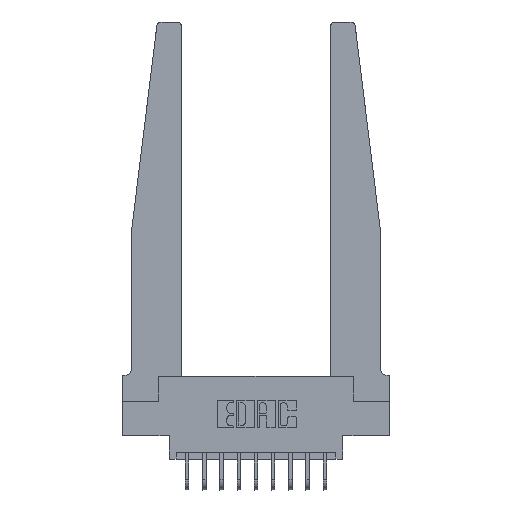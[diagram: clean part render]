
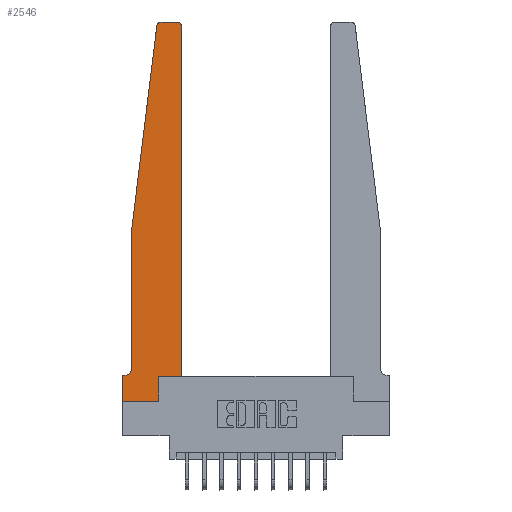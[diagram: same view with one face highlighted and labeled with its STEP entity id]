
A CAD part, top view. The second image highlights one B-rep face of the part: STEP entity #2546.
In plain terms, the highlighted planar face has unit normal (0, 0, 1).
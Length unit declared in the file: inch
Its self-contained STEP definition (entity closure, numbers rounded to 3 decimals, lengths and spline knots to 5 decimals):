
#335 = EDGE_LOOP ( 'NONE', ( #10804, #16728, #8403, #9608, #5358, #16873, #14625, #6112, #15196, #16663, #15041, #6610 ) ) ;
#360 = DIRECTION ( 'NONE',  ( 1., 0., 0. ) ) ;
#439 = DIRECTION ( 'NONE',  ( 0., 0., 1. ) ) ;
#621 = CARTESIAN_POINT ( 'NONE',  ( 0., 0.1875, 0.37 ) ) ;
#931 = EDGE_CURVE ( 'NONE', #7336, #2354, #7570, .T. ) ;
#939 = CARTESIAN_POINT ( 'NONE',  ( 0.065, 1.25, 0.37 ) ) ;
#1289 = VECTOR ( 'NONE', #5804, 39.37008 ) ;
#1539 = CARTESIAN_POINT ( 'NONE',  ( 0.25, 2.75, 0.37 ) ) ;
#1675 = AXIS2_PLACEMENT_3D ( 'NONE', #13910, #439, #15521 ) ;
#1919 = EDGE_CURVE ( 'NONE', #13978, #9623, #15822, .T. ) ;
#2292 = DIRECTION ( 'NONE',  ( 0., 0., -1. ) ) ;
#2296 = CARTESIAN_POINT ( 'NONE',  ( 0.015, 0.1875, 0.37 ) ) ;
#2354 = VERTEX_POINT ( 'NONE', #2296 ) ;
#2460 = EDGE_CURVE ( 'NONE', #5605, #12846, #15492, .T. ) ;
#2537 = DIRECTION ( 'NONE',  ( -0.122, -0.992, 0. ) ) ;
#2546 = ADVANCED_FACE ( 'NONE', ( #13732 ), #3245, .T. ) ;
#2729 = EDGE_CURVE ( 'NONE', #17421, #4041, #17077, .T. ) ;
#2740 = VERTEX_POINT ( 'NONE', #8982 ) ;
#2864 = CARTESIAN_POINT ( 'NONE',  ( 0.2605, 0., 0.37 ) ) ;
#3117 = DIRECTION ( 'NONE',  ( -1., 0., 0. ) ) ;
#3245 = PLANE ( 'NONE',  #6204 ) ;
#3378 = VECTOR ( 'NONE', #5055, 39.37008 ) ;
#3741 = CARTESIAN_POINT ( 'NONE',  ( 0.425, 0.18, 0.37 ) ) ;
#3775 = EDGE_CURVE ( 'NONE', #5778, #13978, #10213, .T. ) ;
#3785 = CARTESIAN_POINT ( 'NONE',  ( 0., 0., 0.37 ) ) ;
#4041 = VERTEX_POINT ( 'NONE', #16283 ) ;
#4111 = DIRECTION ( 'NONE',  ( -1., 0., 0. ) ) ;
#4473 = CARTESIAN_POINT ( 'NONE',  ( 0.395, 2.75, 0.37 ) ) ;
#4482 = CARTESIAN_POINT ( 'NONE',  ( 0.425, 0.18, 0.37 ) ) ;
#5036 = VECTOR ( 'NONE', #10310, 39.37008 ) ;
#5055 = DIRECTION ( 'NONE',  ( 0., -1., 0. ) ) ;
#5325 = EDGE_CURVE ( 'NONE', #12846, #2740, #13802, .T. ) ;
#5356 = VERTEX_POINT ( 'NONE', #14887 ) ;
#5358 = ORIENTED_EDGE ( 'NONE', *, *, #931, .T. ) ;
#5383 = CARTESIAN_POINT ( 'NONE',  ( 0.065, 0.2375, 0.37 ) ) ;
#5605 = VERTEX_POINT ( 'NONE', #11864 ) ;
#5778 = VERTEX_POINT ( 'NONE', #2864 ) ;
#5804 = DIRECTION ( 'NONE',  ( 0., 1., 0. ) ) ;
#5929 = VERTEX_POINT ( 'NONE', #7438 ) ;
#6001 = EDGE_CURVE ( 'NONE', #4041, #7336, #17312, .T. ) ;
#6112 = ORIENTED_EDGE ( 'NONE', *, *, #16059, .T. ) ;
#6204 = AXIS2_PLACEMENT_3D ( 'NONE', #621, #7048, #360 ) ;
#6610 = ORIENTED_EDGE ( 'NONE', *, *, #2460, .T. ) ;
#6832 = CARTESIAN_POINT ( 'NONE',  ( 0.27653, 2.72, 0.37 ) ) ;
#7048 = DIRECTION ( 'NONE',  ( 0., 0., 1. ) ) ;
#7225 = CIRCLE ( 'NONE', #17085, 0.03 ) ;
#7336 = VERTEX_POINT ( 'NONE', #5383 ) ;
#7392 = CARTESIAN_POINT ( 'NONE',  ( 0.425, 0.18, 0.37 ) ) ;
#7438 = CARTESIAN_POINT ( 'NONE',  ( 0., 0., 0.37 ) ) ;
#7570 = CIRCLE ( 'NONE', #8400, 0.05 ) ;
#7676 = DIRECTION ( 'NONE',  ( -1., 0., 0. ) ) ;
#8400 = AXIS2_PLACEMENT_3D ( 'NONE', #10238, #2292, #7676 ) ;
#8403 = ORIENTED_EDGE ( 'NONE', *, *, #2729, .T. ) ;
#8982 = CARTESIAN_POINT ( 'NONE',  ( 0.27653, 2.75, 0.37 ) ) ;
#9178 = VECTOR ( 'NONE', #15874, 39.37008 ) ;
#9466 = DIRECTION ( 'NONE',  ( 0., 0., 1. ) ) ;
#9608 = ORIENTED_EDGE ( 'NONE', *, *, #6001, .T. ) ;
#9623 = VERTEX_POINT ( 'NONE', #4482 ) ;
#9911 = LINE ( 'NONE', #16681, #13357 ) ;
#10213 = LINE ( 'NONE', #14179, #14882 ) ;
#10238 = CARTESIAN_POINT ( 'NONE',  ( 0.015, 0.2375, 0.37 ) ) ;
#10310 = DIRECTION ( 'NONE',  ( 0., -1., 0. ) ) ;
#10499 = CARTESIAN_POINT ( 'NONE',  ( 0., 0., 0.37 ) ) ;
#10608 = CARTESIAN_POINT ( 'NONE',  ( 0.2605, 0.18, 0.37 ) ) ;
#10804 = ORIENTED_EDGE ( 'NONE', *, *, #5325, .T. ) ;
#10983 = VECTOR ( 'NONE', #15564, 39.37008 ) ;
#11339 = EDGE_CURVE ( 'NONE', #5356, #5929, #11895, .T. ) ;
#11864 = CARTESIAN_POINT ( 'NONE',  ( 0.425, 2.72, 0.37 ) ) ;
#11895 = LINE ( 'NONE', #3785, #5036 ) ;
#11939 = DIRECTION ( 'NONE',  ( 1., 0., 0. ) ) ;
#12330 = CARTESIAN_POINT ( 'NONE',  ( 0.24675, 2.72367, 0.37 ) ) ;
#12846 = VERTEX_POINT ( 'NONE', #4473 ) ;
#12855 = LINE ( 'NONE', #7392, #1289 ) ;
#13004 = CARTESIAN_POINT ( 'NONE',  ( 0.065, 1.25, 0.37 ) ) ;
#13357 = VECTOR ( 'NONE', #3117, 39.37008 ) ;
#13712 = EDGE_CURVE ( 'NONE', #2354, #5356, #9911, .T. ) ;
#13732 = FACE_OUTER_BOUND ( 'NONE', #335, .T. ) ;
#13781 = VECTOR ( 'NONE', #2537, 39.37008 ) ;
#13802 = LINE ( 'NONE', #1539, #17190 ) ;
#13910 = CARTESIAN_POINT ( 'NONE',  ( 0.395, 2.72, 0.37 ) ) ;
#13978 = VERTEX_POINT ( 'NONE', #10608 ) ;
#14179 = CARTESIAN_POINT ( 'NONE',  ( 0.2605, 0.18, 0.37 ) ) ;
#14359 = DIRECTION ( 'NONE',  ( 0., 1., 0. ) ) ;
#14625 = ORIENTED_EDGE ( 'NONE', *, *, #11339, .T. ) ;
#14882 = VECTOR ( 'NONE', #14359, 39.37008 ) ;
#14887 = CARTESIAN_POINT ( 'NONE',  ( 0., 0.1875, 0.37 ) ) ;
#15041 = ORIENTED_EDGE ( 'NONE', *, *, #16232, .T. ) ;
#15196 = ORIENTED_EDGE ( 'NONE', *, *, #3775, .T. ) ;
#15492 = CIRCLE ( 'NONE', #1675, 0.03 ) ;
#15521 = DIRECTION ( 'NONE',  ( 1., 0., 0. ) ) ;
#15564 = DIRECTION ( 'NONE',  ( 1., 0., 0. ) ) ;
#15822 = LINE ( 'NONE', #3741, #10983 ) ;
#15874 = DIRECTION ( 'NONE',  ( 1., 0., 0. ) ) ;
#16059 = EDGE_CURVE ( 'NONE', #5929, #5778, #17210, .T. ) ;
#16232 = EDGE_CURVE ( 'NONE', #9623, #5605, #12855, .T. ) ;
#16283 = CARTESIAN_POINT ( 'NONE',  ( 0.065, 1.25, 0.37 ) ) ;
#16663 = ORIENTED_EDGE ( 'NONE', *, *, #1919, .T. ) ;
#16681 = CARTESIAN_POINT ( 'NONE',  ( 0.065, 0.1875, 0.37 ) ) ;
#16728 = ORIENTED_EDGE ( 'NONE', *, *, #16965, .T. ) ;
#16873 = ORIENTED_EDGE ( 'NONE', *, *, #13712, .T. ) ;
#16965 = EDGE_CURVE ( 'NONE', #2740, #17421, #7225, .T. ) ;
#17077 = LINE ( 'NONE', #939, #13781 ) ;
#17085 = AXIS2_PLACEMENT_3D ( 'NONE', #6832, #9466, #11939 ) ;
#17190 = VECTOR ( 'NONE', #4111, 39.37008 ) ;
#17210 = LINE ( 'NONE', #10499, #9178 ) ;
#17312 = LINE ( 'NONE', #13004, #3378 ) ;
#17421 = VERTEX_POINT ( 'NONE', #12330 ) ;
